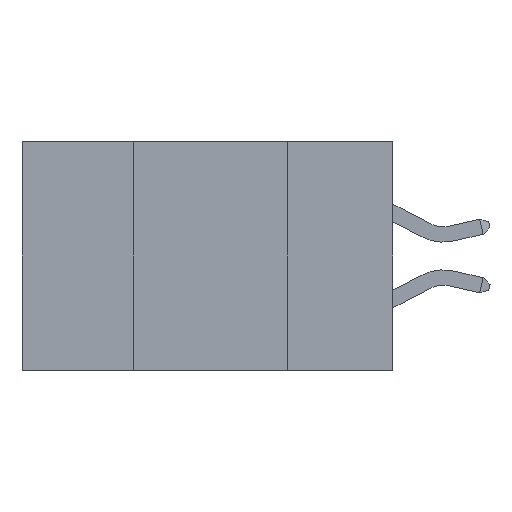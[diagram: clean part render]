
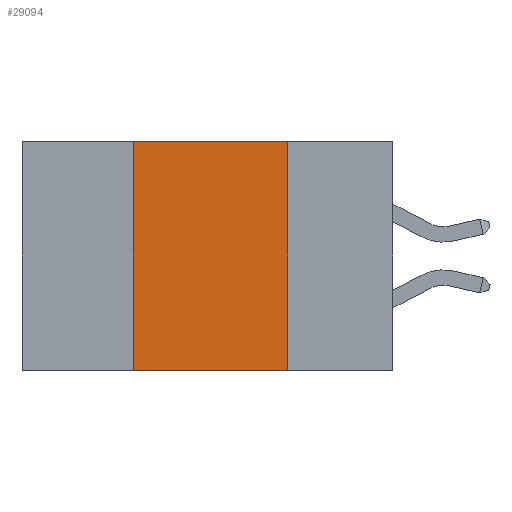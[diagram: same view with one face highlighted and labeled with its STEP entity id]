
A CAD part, left-side view. The second image highlights one B-rep face of the part: STEP entity #29094.
In plain terms, the highlighted planar face has unit normal (-1, 0, 0).
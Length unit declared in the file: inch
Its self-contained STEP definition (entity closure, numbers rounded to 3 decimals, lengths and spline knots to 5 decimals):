
#1295 = DIRECTION ( 'NONE',  ( 0., 0., 1. ) ) ;
#1305 = VERTEX_POINT ( 'NONE', #12976 ) ;
#1355 = VECTOR ( 'NONE', #24779, 39.37008 ) ;
#1942 = DIRECTION ( 'NONE',  ( 0., 0., -1. ) ) ;
#2231 = VECTOR ( 'NONE', #1295, 39.37008 ) ;
#2961 = AXIS2_PLACEMENT_3D ( 'NONE', #15265, #41476, #1942 ) ;
#3015 = ORIENTED_EDGE ( 'NONE', *, *, #10617, .F. ) ;
#3042 = LINE ( 'NONE', #33197, #15879 ) ;
#3199 = ORIENTED_EDGE ( 'NONE', *, *, #4680, .F. ) ;
#4680 = EDGE_CURVE ( 'NONE', #8581, #18558, #19690, .T. ) ;
#4694 = CARTESIAN_POINT ( 'NONE',  ( 0., 0.17, 0. ) ) ;
#8581 = VERTEX_POINT ( 'NONE', #25283 ) ;
#8890 = FACE_OUTER_BOUND ( 'NONE', #11966, .T. ) ;
#10617 = EDGE_CURVE ( 'NONE', #18558, #31385, #28527, .T. ) ;
#11966 = EDGE_LOOP ( 'NONE', ( #36010, #3015, #3199, #37897 ) ) ;
#12976 = CARTESIAN_POINT ( 'NONE',  ( 0., 0.17, -0.37 ) ) ;
#15265 = CARTESIAN_POINT ( 'NONE',  ( 0., 0.6, 0. ) ) ;
#15879 = VECTOR ( 'NONE', #19882, 39.37008 ) ;
#16207 = CARTESIAN_POINT ( 'NONE',  ( 0., 0.42, 0. ) ) ;
#16280 = VECTOR ( 'NONE', #17744, 39.37008 ) ;
#17744 = DIRECTION ( 'NONE',  ( 0., 0., -1. ) ) ;
#18558 = VERTEX_POINT ( 'NONE', #16207 ) ;
#18792 = EDGE_CURVE ( 'NONE', #31385, #1305, #36768, .T. ) ;
#19690 = LINE ( 'NONE', #31059, #2231 ) ;
#19882 = DIRECTION ( 'NONE',  ( 0., -1., 0. ) ) ;
#21271 = CARTESIAN_POINT ( 'NONE',  ( 0., 0.17, 0. ) ) ;
#24779 = DIRECTION ( 'NONE',  ( 0., -1., 0. ) ) ;
#25283 = CARTESIAN_POINT ( 'NONE',  ( 0., 0.42, -0.37 ) ) ;
#28527 = LINE ( 'NONE', #31670, #1355 ) ;
#29094 = ADVANCED_FACE ( 'NONE', ( #8890 ), #31281, .F. ) ;
#31059 = CARTESIAN_POINT ( 'NONE',  ( 0., 0.42, 0. ) ) ;
#31176 = EDGE_CURVE ( 'NONE', #8581, #1305, #3042, .T. ) ;
#31281 = PLANE ( 'NONE',  #2961 ) ;
#31385 = VERTEX_POINT ( 'NONE', #21271 ) ;
#31670 = CARTESIAN_POINT ( 'NONE',  ( 0., 0.6, 0. ) ) ;
#33197 = CARTESIAN_POINT ( 'NONE',  ( 0., 0.6, -0.37 ) ) ;
#36010 = ORIENTED_EDGE ( 'NONE', *, *, #18792, .F. ) ;
#36768 = LINE ( 'NONE', #4694, #16280 ) ;
#37897 = ORIENTED_EDGE ( 'NONE', *, *, #31176, .T. ) ;
#41476 = DIRECTION ( 'NONE',  ( 1., 0., 0. ) ) ;
